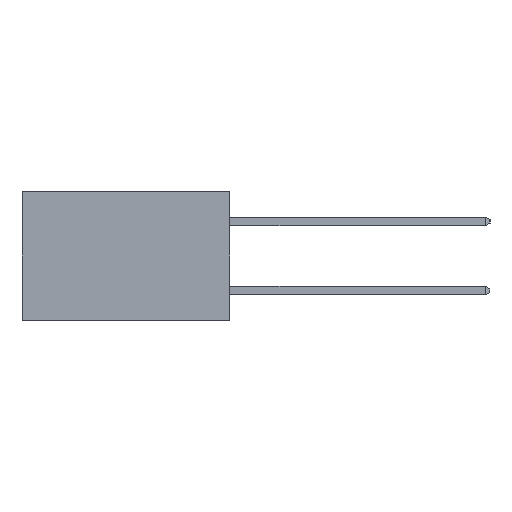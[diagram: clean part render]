
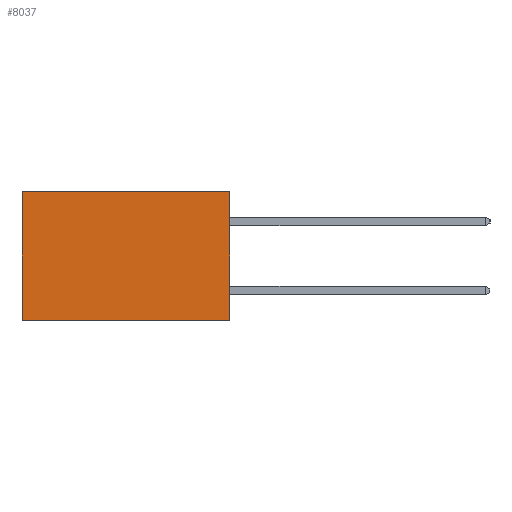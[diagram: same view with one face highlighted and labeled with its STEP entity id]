
A CAD part, left-side view. The second image highlights one B-rep face of the part: STEP entity #8037.
In plain terms, the highlighted planar face has unit normal (-1, 0, 0).
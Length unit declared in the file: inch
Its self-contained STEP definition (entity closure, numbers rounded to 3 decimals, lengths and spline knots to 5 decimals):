
#1251 = EDGE_LOOP ( 'NONE', ( #10637, #2365, #14872, #17614 ) ) ;
#2365 = ORIENTED_EDGE ( 'NONE', *, *, #16169, .F. ) ;
#3786 = EDGE_CURVE ( 'NONE', #15993, #20882, #7085, .T. ) ;
#4270 = FACE_OUTER_BOUND ( 'NONE', #1251, .T. ) ;
#5420 = EDGE_CURVE ( 'NONE', #20882, #7814, #14489, .T. ) ;
#5777 = DIRECTION ( 'NONE',  ( 0., 0., -1. ) ) ;
#5913 = VECTOR ( 'NONE', #11853, 39.37008 ) ;
#7085 = LINE ( 'NONE', #14118, #5913 ) ;
#7814 = VERTEX_POINT ( 'NONE', #16881 ) ;
#8037 = ADVANCED_FACE ( 'NONE', ( #4270 ), #11836, .F. ) ;
#8071 = LINE ( 'NONE', #13888, #12661 ) ;
#8095 = CARTESIAN_POINT ( 'NONE',  ( 0.298, 0., -0.37 ) ) ;
#9084 = CARTESIAN_POINT ( 'NONE',  ( 0.298, 0.6, 0. ) ) ;
#10105 = DIRECTION ( 'NONE',  ( 0., 0., -1. ) ) ;
#10574 = VERTEX_POINT ( 'NONE', #8095 ) ;
#10637 = ORIENTED_EDGE ( 'NONE', *, *, #5420, .T. ) ;
#10663 = AXIS2_PLACEMENT_3D ( 'NONE', #19164, #20959, #10105 ) ;
#11284 = VECTOR ( 'NONE', #22050, 39.37008 ) ;
#11836 = PLANE ( 'NONE',  #10663 ) ;
#11853 = DIRECTION ( 'NONE',  ( 0., 1., 0. ) ) ;
#12661 = VECTOR ( 'NONE', #17583, 39.37008 ) ;
#13888 = CARTESIAN_POINT ( 'NONE',  ( 0.298, 0., -0.37 ) ) ;
#14118 = CARTESIAN_POINT ( 'NONE',  ( 0.298, 0., 0. ) ) ;
#14489 = LINE ( 'NONE', #9084, #23462 ) ;
#14872 = ORIENTED_EDGE ( 'NONE', *, *, #23259, .F. ) ;
#15264 = CARTESIAN_POINT ( 'NONE',  ( 0.298, 0., 0. ) ) ;
#15993 = VERTEX_POINT ( 'NONE', #15264 ) ;
#16169 = EDGE_CURVE ( 'NONE', #10574, #7814, #8071, .T. ) ;
#16881 = CARTESIAN_POINT ( 'NONE',  ( 0.298, 0.6, -0.37 ) ) ;
#17583 = DIRECTION ( 'NONE',  ( 0., 1., 0. ) ) ;
#17614 = ORIENTED_EDGE ( 'NONE', *, *, #3786, .T. ) ;
#18555 = CARTESIAN_POINT ( 'NONE',  ( 0.298, 0.6, 0. ) ) ;
#19164 = CARTESIAN_POINT ( 'NONE',  ( 0.298, 0., 0. ) ) ;
#20376 = LINE ( 'NONE', #20424, #11284 ) ;
#20424 = CARTESIAN_POINT ( 'NONE',  ( 0.298, 0., 0. ) ) ;
#20882 = VERTEX_POINT ( 'NONE', #18555 ) ;
#20959 = DIRECTION ( 'NONE',  ( 1., 0., 0. ) ) ;
#22050 = DIRECTION ( 'NONE',  ( 0., 0., -1. ) ) ;
#23259 = EDGE_CURVE ( 'NONE', #15993, #10574, #20376, .T. ) ;
#23462 = VECTOR ( 'NONE', #5777, 39.37008 ) ;
